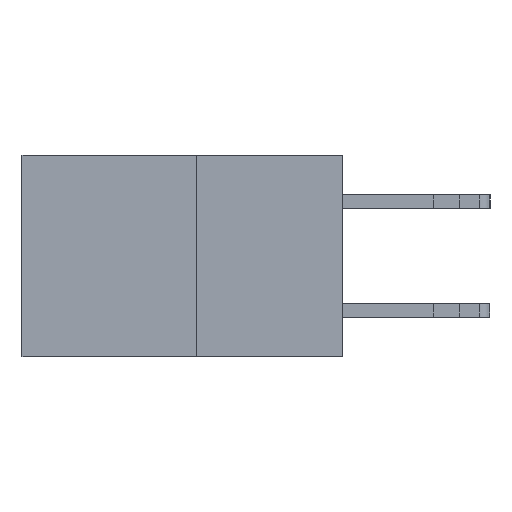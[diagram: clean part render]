
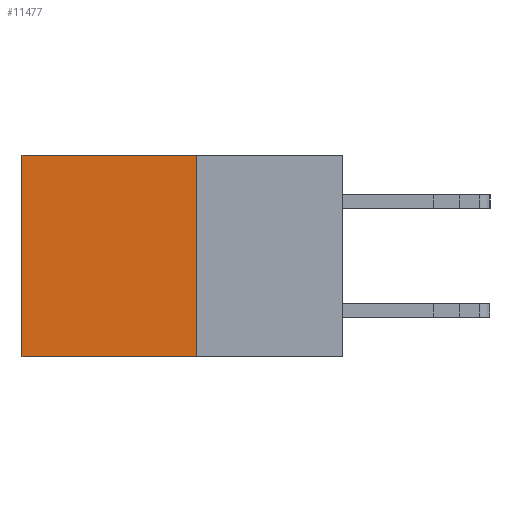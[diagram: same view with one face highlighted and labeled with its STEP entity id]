
A CAD part, left-side view. The second image highlights one B-rep face of the part: STEP entity #11477.
In plain terms, the highlighted planar face has unit normal (-1, 0, 0).
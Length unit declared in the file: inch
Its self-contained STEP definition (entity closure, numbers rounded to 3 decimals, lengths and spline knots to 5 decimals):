
#228 = EDGE_CURVE ( 'NONE', #7436, #12398, #24701, .T. ) ;
#1996 = LINE ( 'NONE', #10267, #12476 ) ;
#2344 = ORIENTED_EDGE ( 'NONE', *, *, #7847, .T. ) ;
#4701 = LINE ( 'NONE', #5520, #21292 ) ;
#5520 = CARTESIAN_POINT ( 'NONE',  ( 0.277, 0.27, 0. ) ) ;
#6135 = VERTEX_POINT ( 'NONE', #12543 ) ;
#7430 = DIRECTION ( 'NONE',  ( 0., 1., 0. ) ) ;
#7436 = VERTEX_POINT ( 'NONE', #25862 ) ;
#7847 = EDGE_CURVE ( 'NONE', #6135, #12398, #1996, .T. ) ;
#8014 = CARTESIAN_POINT ( 'NONE',  ( 0.277, 0.27, -0.37 ) ) ;
#9034 = CARTESIAN_POINT ( 'NONE',  ( 0.277, 0.59, -0.37 ) ) ;
#9173 = VECTOR ( 'NONE', #17869, 39.37008 ) ;
#9514 = DIRECTION ( 'NONE',  ( 0., 0., -1. ) ) ;
#9692 = DIRECTION ( 'NONE',  ( 0., 0., -1. ) ) ;
#10267 = CARTESIAN_POINT ( 'NONE',  ( 0.277, 0.59, -0.37 ) ) ;
#10978 = EDGE_CURVE ( 'NONE', #24163, #6135, #4701, .T. ) ;
#11477 = ADVANCED_FACE ( 'NONE', ( #18707 ), #19886, .F. ) ;
#11564 = CARTESIAN_POINT ( 'NONE',  ( 0.277, 0.27, -0.37 ) ) ;
#12398 = VERTEX_POINT ( 'NONE', #9034 ) ;
#12476 = VECTOR ( 'NONE', #9692, 39.37008 ) ;
#12543 = CARTESIAN_POINT ( 'NONE',  ( 0.277, 0.59, 0. ) ) ;
#12861 = CARTESIAN_POINT ( 'NONE',  ( 0.277, 0.27, 0. ) ) ;
#13029 = VECTOR ( 'NONE', #7430, 39.37008 ) ;
#13134 = EDGE_CURVE ( 'NONE', #24163, #7436, #22171, .T. ) ;
#15750 = CARTESIAN_POINT ( 'NONE',  ( 0.277, 0.27, -0.37 ) ) ;
#17054 = ORIENTED_EDGE ( 'NONE', *, *, #10978, .T. ) ;
#17869 = DIRECTION ( 'NONE',  ( 0., 0., -1. ) ) ;
#18707 = FACE_OUTER_BOUND ( 'NONE', #21796, .T. ) ;
#19886 = PLANE ( 'NONE',  #26618 ) ;
#21292 = VECTOR ( 'NONE', #26233, 39.37008 ) ;
#21796 = EDGE_LOOP ( 'NONE', ( #2344, #22626, #25733, #17054 ) ) ;
#21949 = DIRECTION ( 'NONE',  ( 1., 0., 0. ) ) ;
#22171 = LINE ( 'NONE', #11564, #9173 ) ;
#22626 = ORIENTED_EDGE ( 'NONE', *, *, #228, .F. ) ;
#24163 = VERTEX_POINT ( 'NONE', #12861 ) ;
#24701 = LINE ( 'NONE', #8014, #13029 ) ;
#25733 = ORIENTED_EDGE ( 'NONE', *, *, #13134, .F. ) ;
#25862 = CARTESIAN_POINT ( 'NONE',  ( 0.277, 0.27, -0.37 ) ) ;
#26233 = DIRECTION ( 'NONE',  ( 0., 1., 0. ) ) ;
#26618 = AXIS2_PLACEMENT_3D ( 'NONE', #15750, #21949, #9514 ) ;
